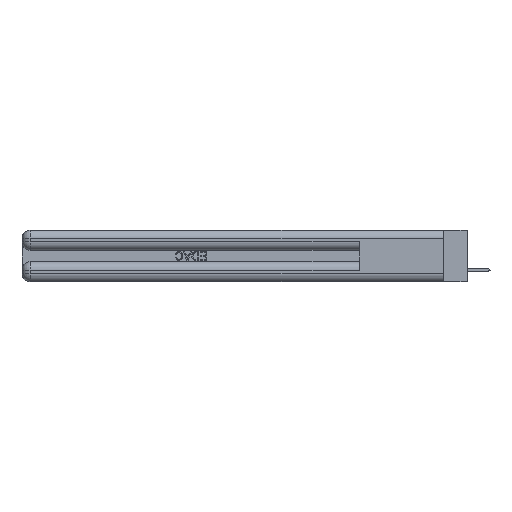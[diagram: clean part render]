
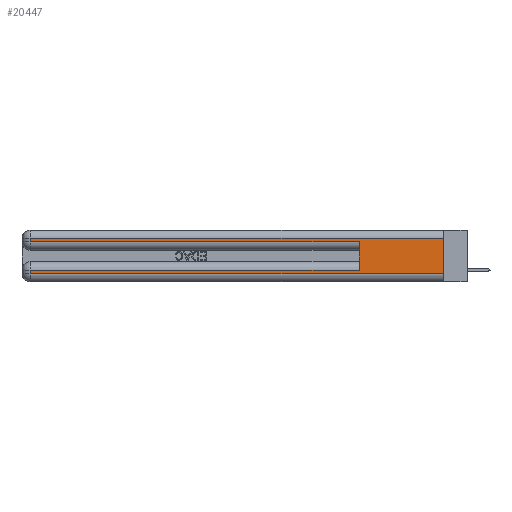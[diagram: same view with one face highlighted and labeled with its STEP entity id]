
A CAD part, left-side view. The second image highlights one B-rep face of the part: STEP entity #20447.
In plain terms, the highlighted planar face has unit normal (-1, 0, 0).
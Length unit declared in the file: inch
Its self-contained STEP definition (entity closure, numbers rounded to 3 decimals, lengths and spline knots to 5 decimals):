
#518 = CARTESIAN_POINT ( 'NONE',  ( 0., 0., 0.285 ) ) ;
#1140 = CARTESIAN_POINT ( 'NONE',  ( 0., 2.94, 0.285 ) ) ;
#1897 = VECTOR ( 'NONE', #20564, 39.37008 ) ;
#2820 = CARTESIAN_POINT ( 'NONE',  ( 0., 0.6, 0.085 ) ) ;
#2896 = VECTOR ( 'NONE', #11616, 39.37008 ) ;
#4979 = VECTOR ( 'NONE', #48793, 39.37008 ) ;
#5798 = CARTESIAN_POINT ( 'NONE',  ( 0., 2.94, 0.085 ) ) ;
#5870 = CARTESIAN_POINT ( 'NONE',  ( 0., 0., 0.085 ) ) ;
#7185 = VERTEX_POINT ( 'NONE', #33134 ) ;
#7407 = DIRECTION ( 'NONE',  ( 1., 0., 0. ) ) ;
#7926 = CARTESIAN_POINT ( 'NONE',  ( 0., 0., 0.37 ) ) ;
#8093 = CARTESIAN_POINT ( 'NONE',  ( 0., 2.94, 0.37 ) ) ;
#8544 = VERTEX_POINT ( 'NONE', #33183 ) ;
#9081 = EDGE_CURVE ( 'NONE', #14019, #48106, #41477, .T. ) ;
#9874 = ORIENTED_EDGE ( 'NONE', *, *, #32787, .T. ) ;
#10352 = EDGE_CURVE ( 'NONE', #25491, #8544, #25236, .T. ) ;
#11297 = ORIENTED_EDGE ( 'NONE', *, *, #46624, .F. ) ;
#11616 = DIRECTION ( 'NONE',  ( 0., 0., -1. ) ) ;
#12620 = CARTESIAN_POINT ( 'NONE',  ( 0., 2.94, 0.31 ) ) ;
#12628 = AXIS2_PLACEMENT_3D ( 'NONE', #33096, #7407, #38341 ) ;
#13441 = CARTESIAN_POINT ( 'NONE',  ( 0., 2.94, 0.06 ) ) ;
#13806 = VERTEX_POINT ( 'NONE', #1140 ) ;
#14019 = VERTEX_POINT ( 'NONE', #2820 ) ;
#14767 = ORIENTED_EDGE ( 'NONE', *, *, #9081, .T. ) ;
#15875 = VECTOR ( 'NONE', #25255, 39.37008 ) ;
#16972 = VECTOR ( 'NONE', #31240, 39.37008 ) ;
#17123 = LINE ( 'NONE', #36909, #15875 ) ;
#18587 = LINE ( 'NONE', #32723, #47817 ) ;
#18721 = ORIENTED_EDGE ( 'NONE', *, *, #46586, .T. ) ;
#18842 = CARTESIAN_POINT ( 'NONE',  ( 0., 2.94, 0.37 ) ) ;
#19379 = ORIENTED_EDGE ( 'NONE', *, *, #10352, .T. ) ;
#19391 = CARTESIAN_POINT ( 'NONE',  ( 0., 0., 0.06 ) ) ;
#20072 = EDGE_LOOP ( 'NONE', ( #11297, #25618, #23644, #9874, #33947, #14767, #18721, #19379 ) ) ;
#20447 = ADVANCED_FACE ( 'NONE', ( #39697 ), #37426, .F. ) ;
#20564 = DIRECTION ( 'NONE',  ( 0., -1., 0. ) ) ;
#20614 = LINE ( 'NONE', #18842, #4979 ) ;
#21396 = LINE ( 'NONE', #8093, #30868 ) ;
#23234 = VERTEX_POINT ( 'NONE', #12620 ) ;
#23644 = ORIENTED_EDGE ( 'NONE', *, *, #31105, .T. ) ;
#23895 = CARTESIAN_POINT ( 'NONE',  ( 0., 0.6, 0.285 ) ) ;
#25236 = LINE ( 'NONE', #19391, #1897 ) ;
#25255 = DIRECTION ( 'NONE',  ( 0., 1., 0. ) ) ;
#25491 = VERTEX_POINT ( 'NONE', #13441 ) ;
#25618 = ORIENTED_EDGE ( 'NONE', *, *, #31319, .T. ) ;
#26386 = DIRECTION ( 'NONE',  ( 0., 0., 1. ) ) ;
#27081 = LINE ( 'NONE', #518, #16972 ) ;
#27944 = LINE ( 'NONE', #7926, #2896 ) ;
#28863 = EDGE_CURVE ( 'NONE', #14019, #33822, #18587, .T. ) ;
#30868 = VECTOR ( 'NONE', #42459, 39.37008 ) ;
#31105 = EDGE_CURVE ( 'NONE', #23234, #13806, #21396, .T. ) ;
#31240 = DIRECTION ( 'NONE',  ( 0., -1., 0. ) ) ;
#31249 = VECTOR ( 'NONE', #47242, 39.37008 ) ;
#31319 = EDGE_CURVE ( 'NONE', #7185, #23234, #17123, .T. ) ;
#32723 = CARTESIAN_POINT ( 'NONE',  ( 0., 0.6, 0.145 ) ) ;
#32787 = EDGE_CURVE ( 'NONE', #13806, #33822, #27081, .T. ) ;
#33096 = CARTESIAN_POINT ( 'NONE',  ( 0., 0., 0.37 ) ) ;
#33134 = CARTESIAN_POINT ( 'NONE',  ( 0., 0., 0.31 ) ) ;
#33183 = CARTESIAN_POINT ( 'NONE',  ( 0., 0., 0.06 ) ) ;
#33822 = VERTEX_POINT ( 'NONE', #23895 ) ;
#33947 = ORIENTED_EDGE ( 'NONE', *, *, #28863, .F. ) ;
#36909 = CARTESIAN_POINT ( 'NONE',  ( 0., 0., 0.31 ) ) ;
#37426 = PLANE ( 'NONE',  #12628 ) ;
#38341 = DIRECTION ( 'NONE',  ( 0., 0., -1. ) ) ;
#39697 = FACE_OUTER_BOUND ( 'NONE', #20072, .T. ) ;
#41477 = LINE ( 'NONE', #5870, #31249 ) ;
#42459 = DIRECTION ( 'NONE',  ( 0., 0., -1. ) ) ;
#46586 = EDGE_CURVE ( 'NONE', #48106, #25491, #20614, .T. ) ;
#46624 = EDGE_CURVE ( 'NONE', #7185, #8544, #27944, .T. ) ;
#47242 = DIRECTION ( 'NONE',  ( 0., 1., 0. ) ) ;
#47817 = VECTOR ( 'NONE', #26386, 39.37008 ) ;
#48106 = VERTEX_POINT ( 'NONE', #5798 ) ;
#48793 = DIRECTION ( 'NONE',  ( 0., 0., -1. ) ) ;
